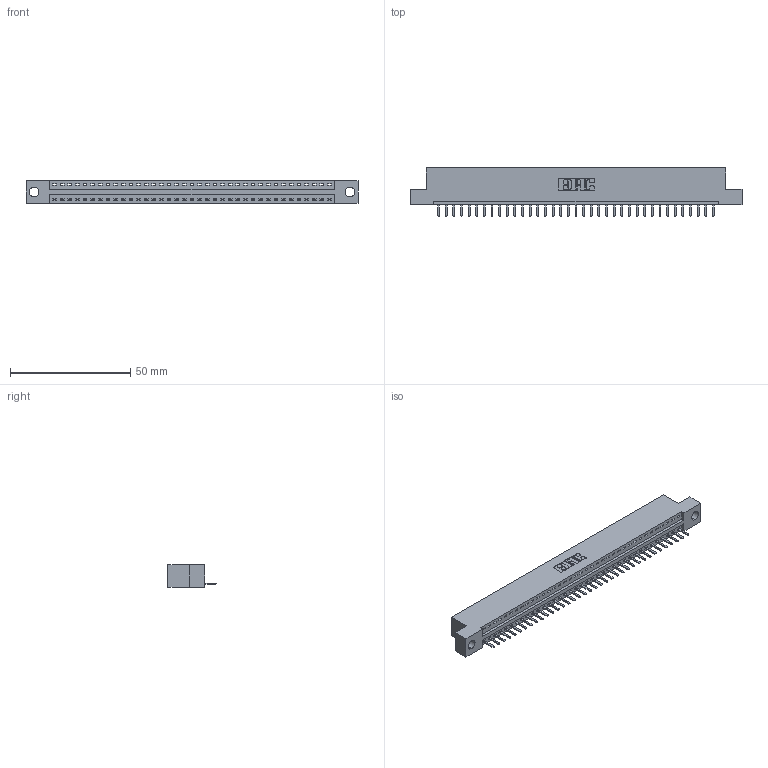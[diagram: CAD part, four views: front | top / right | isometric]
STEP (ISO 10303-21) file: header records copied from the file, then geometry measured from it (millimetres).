
FILE_DESCRIPTION (( 'STEP AP203' ), '1' );
FILE_NAME ('346-037-520-104.STEP', '2022-05-07T02:09:23', ( '' ), ( '' ), 'SwSTEP 2.0', 'SolidWorks 2020', '' );
FILE_SCHEMA (( 'CONFIG_CONTROL_DESIGN' ));
Length unit declared in the file: inch
Products named in the file (3): 346-037-520-104; 346 Part_Flush Mounting Lugs - 0.156 Dia-TH; 345-292-001_345-293-120
Assembly tree (38 placements, depth 2):
  346-037-520-104
    346 Part_Flush Mounting Lugs - 0.156 Dia-TH
    345-292-001_345-293-120  x37
Bounding box: 138.05 x 20.02 x 9.4 mm (x, y, z)
Volume: 12967.5 mm3; surface area: 15635.7 mm2
Topology: 38 solids, 38 shells, 2430 faces, 7173 edges, 4682 vertices
Faces by surface type: plane 1644, cylinder 786
Entity records: 24169 total; most frequent: CARTESIAN_POINT 4165, ORIENTED_EDGE 4122, DIRECTION 3667, EDGE_CURVE 2061, VECTOR 1777, LINE 1777, VERTEX_POINT 1370, AXIS2_PLACEMENT_3D 945
